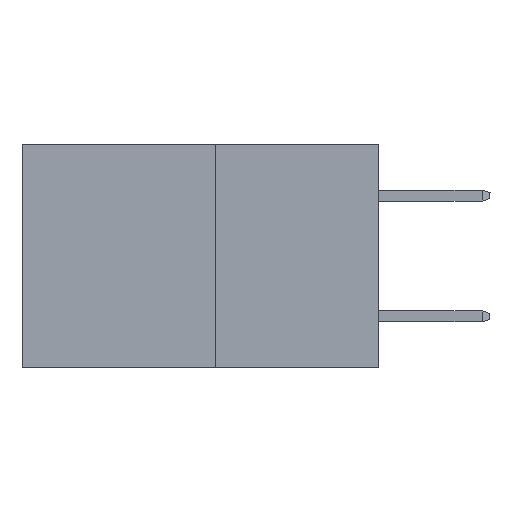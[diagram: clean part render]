
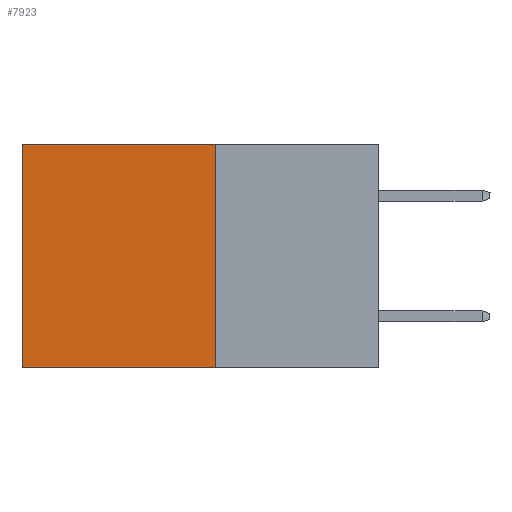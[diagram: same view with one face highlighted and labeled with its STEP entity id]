
A CAD part, left-side view. The second image highlights one B-rep face of the part: STEP entity #7923.
In plain terms, the highlighted planar face has unit normal (-1, 0, 0).
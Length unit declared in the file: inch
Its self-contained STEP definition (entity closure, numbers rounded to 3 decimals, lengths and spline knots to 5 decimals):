
#815 = CARTESIAN_POINT ( 'NONE',  ( 0.277, 0.59, -0.37 ) ) ;
#1553 = VERTEX_POINT ( 'NONE', #815 ) ;
#2214 = ORIENTED_EDGE ( 'NONE', *, *, #2321, .F. ) ;
#2321 = EDGE_CURVE ( 'NONE', #13661, #1553, #11255, .T. ) ;
#2705 = VECTOR ( 'NONE', #17691, 39.37008 ) ;
#3276 = ORIENTED_EDGE ( 'NONE', *, *, #10291, .F. ) ;
#3412 = DIRECTION ( 'NONE',  ( 0., 0., -1. ) ) ;
#3444 = CARTESIAN_POINT ( 'NONE',  ( 0.277, 0.27, -0.37 ) ) ;
#3793 = EDGE_CURVE ( 'NONE', #10191, #1553, #6445, .T. ) ;
#4334 = CARTESIAN_POINT ( 'NONE',  ( 0.277, 0.27, 0. ) ) ;
#4881 = CARTESIAN_POINT ( 'NONE',  ( 0.277, 0.27, -0.37 ) ) ;
#5014 = CARTESIAN_POINT ( 'NONE',  ( 0.277, 0.59, 0. ) ) ;
#5152 = AXIS2_PLACEMENT_3D ( 'NONE', #13126, #13370, #13358 ) ;
#5405 = LINE ( 'NONE', #4334, #9126 ) ;
#6119 = VERTEX_POINT ( 'NONE', #18772 ) ;
#6259 = DIRECTION ( 'NONE',  ( 0., 1., 0. ) ) ;
#6445 = LINE ( 'NONE', #7771, #2705 ) ;
#6813 = DIRECTION ( 'NONE',  ( 0., 1., 0. ) ) ;
#7771 = CARTESIAN_POINT ( 'NONE',  ( 0.277, 0.59, -0.37 ) ) ;
#7923 = ADVANCED_FACE ( 'NONE', ( #13153 ), #14377, .F. ) ;
#9126 = VECTOR ( 'NONE', #6259, 39.37008 ) ;
#10070 = LINE ( 'NONE', #3444, #18460 ) ;
#10191 = VERTEX_POINT ( 'NONE', #5014 ) ;
#10291 = EDGE_CURVE ( 'NONE', #6119, #13661, #10070, .T. ) ;
#11255 = LINE ( 'NONE', #16029, #19068 ) ;
#13126 = CARTESIAN_POINT ( 'NONE',  ( 0.277, 0.27, -0.37 ) ) ;
#13153 = FACE_OUTER_BOUND ( 'NONE', #15458, .T. ) ;
#13287 = ORIENTED_EDGE ( 'NONE', *, *, #13583, .T. ) ;
#13358 = DIRECTION ( 'NONE',  ( 0., 0., -1. ) ) ;
#13370 = DIRECTION ( 'NONE',  ( 1., 0., 0. ) ) ;
#13583 = EDGE_CURVE ( 'NONE', #6119, #10191, #5405, .T. ) ;
#13661 = VERTEX_POINT ( 'NONE', #4881 ) ;
#14377 = PLANE ( 'NONE',  #5152 ) ;
#14532 = ORIENTED_EDGE ( 'NONE', *, *, #3793, .T. ) ;
#15458 = EDGE_LOOP ( 'NONE', ( #14532, #2214, #3276, #13287 ) ) ;
#16029 = CARTESIAN_POINT ( 'NONE',  ( 0.277, 0.27, -0.37 ) ) ;
#17691 = DIRECTION ( 'NONE',  ( 0., 0., -1. ) ) ;
#18460 = VECTOR ( 'NONE', #3412, 39.37008 ) ;
#18772 = CARTESIAN_POINT ( 'NONE',  ( 0.277, 0.27, 0. ) ) ;
#19068 = VECTOR ( 'NONE', #6813, 39.37008 ) ;
